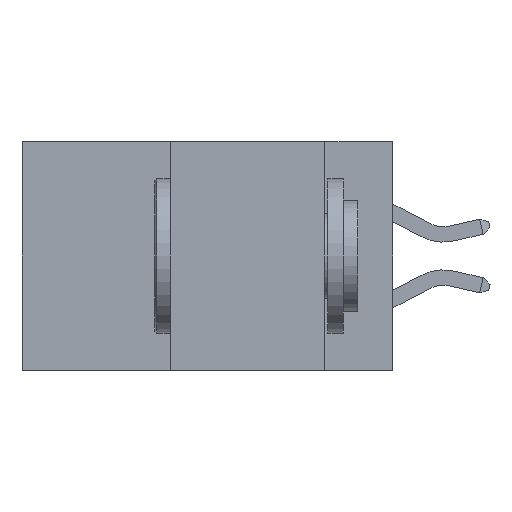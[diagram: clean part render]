
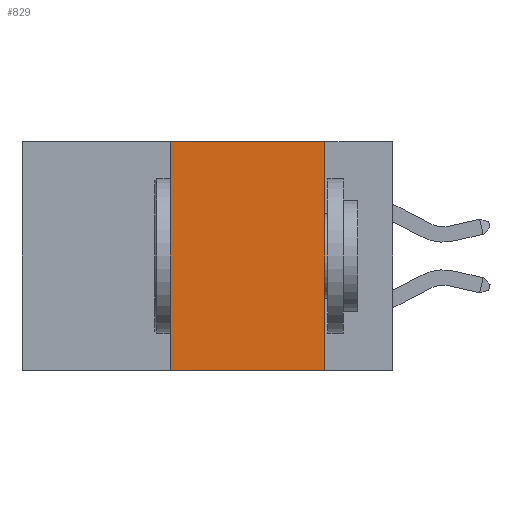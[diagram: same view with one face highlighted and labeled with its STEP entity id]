
A CAD part, left-side view. The second image highlights one B-rep face of the part: STEP entity #829.
In plain terms, the highlighted planar face has unit normal (-1, 0, 0).
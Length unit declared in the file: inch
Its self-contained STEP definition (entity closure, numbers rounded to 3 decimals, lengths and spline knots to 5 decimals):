
#829 = ADVANCED_FACE ( 'NONE', ( #21382 ), #9708, .F. ) ;
#2102 = ORIENTED_EDGE ( 'NONE', *, *, #14431, .T. ) ;
#2536 = DIRECTION ( 'NONE',  ( 0., -1., 0. ) ) ;
#2870 = CARTESIAN_POINT ( 'NONE',  ( 0., 0.11, 0. ) ) ;
#2908 = LINE ( 'NONE', #11422, #21191 ) ;
#3216 = ORIENTED_EDGE ( 'NONE', *, *, #15841, .F. ) ;
#3411 = VERTEX_POINT ( 'NONE', #8428 ) ;
#4402 = DIRECTION ( 'NONE',  ( 0., -1., 0. ) ) ;
#4488 = CARTESIAN_POINT ( 'NONE',  ( 0., 0.6, -0.37 ) ) ;
#4963 = DIRECTION ( 'NONE',  ( 1., 0., 0. ) ) ;
#5495 = DIRECTION ( 'NONE',  ( 0., 0., 1. ) ) ;
#7457 = ORIENTED_EDGE ( 'NONE', *, *, #8247, .F. ) ;
#8247 = EDGE_CURVE ( 'NONE', #8781, #3411, #13745, .T. ) ;
#8428 = CARTESIAN_POINT ( 'NONE',  ( 0., 0.36, 0. ) ) ;
#8709 = ORIENTED_EDGE ( 'NONE', *, *, #15734, .F. ) ;
#8781 = VERTEX_POINT ( 'NONE', #13684 ) ;
#9513 = VECTOR ( 'NONE', #15803, 39.37008 ) ;
#9708 = PLANE ( 'NONE',  #10228 ) ;
#10228 = AXIS2_PLACEMENT_3D ( 'NONE', #14594, #4963, #15607 ) ;
#10327 = CARTESIAN_POINT ( 'NONE',  ( 0., 0.36, 0. ) ) ;
#10643 = VECTOR ( 'NONE', #5495, 39.37008 ) ;
#11267 = VERTEX_POINT ( 'NONE', #2870 ) ;
#11422 = CARTESIAN_POINT ( 'NONE',  ( 0., 0.6, 0. ) ) ;
#12023 = LINE ( 'NONE', #17837, #9513 ) ;
#12181 = CARTESIAN_POINT ( 'NONE',  ( 0., 0.11, -0.37 ) ) ;
#12195 = LINE ( 'NONE', #4488, #21918 ) ;
#13684 = CARTESIAN_POINT ( 'NONE',  ( 0., 0.36, -0.37 ) ) ;
#13745 = LINE ( 'NONE', #10327, #10643 ) ;
#14431 = EDGE_CURVE ( 'NONE', #8781, #19711, #12195, .T. ) ;
#14594 = CARTESIAN_POINT ( 'NONE',  ( 0., 0.6, 0. ) ) ;
#15607 = DIRECTION ( 'NONE',  ( 0., 0., -1. ) ) ;
#15734 = EDGE_CURVE ( 'NONE', #11267, #19711, #12023, .T. ) ;
#15803 = DIRECTION ( 'NONE',  ( 0., 0., -1. ) ) ;
#15841 = EDGE_CURVE ( 'NONE', #3411, #11267, #2908, .T. ) ;
#17837 = CARTESIAN_POINT ( 'NONE',  ( 0., 0.11, 0. ) ) ;
#19711 = VERTEX_POINT ( 'NONE', #12181 ) ;
#21191 = VECTOR ( 'NONE', #4402, 39.37008 ) ;
#21382 = FACE_OUTER_BOUND ( 'NONE', #22791, .T. ) ;
#21918 = VECTOR ( 'NONE', #2536, 39.37008 ) ;
#22791 = EDGE_LOOP ( 'NONE', ( #8709, #3216, #7457, #2102 ) ) ;
